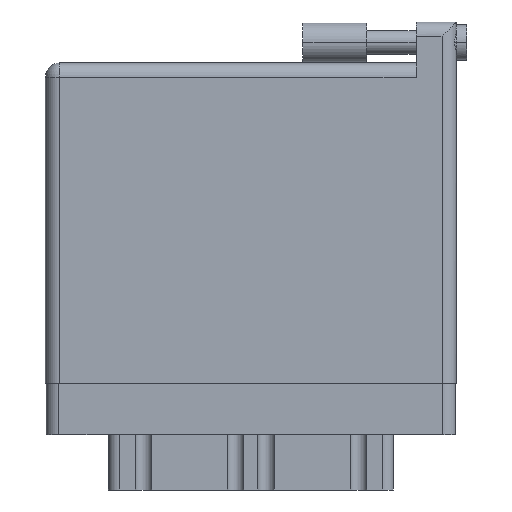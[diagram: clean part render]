
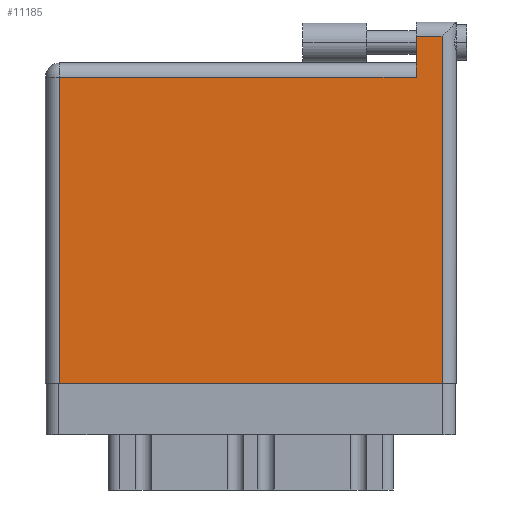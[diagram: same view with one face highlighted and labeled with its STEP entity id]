
A CAD part, front view. The second image highlights one B-rep face of the part: STEP entity #11185.
In plain terms, the highlighted face is planar.
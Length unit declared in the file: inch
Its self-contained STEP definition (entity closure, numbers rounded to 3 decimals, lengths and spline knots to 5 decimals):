
#1038 = CARTESIAN_POINT ( 'NONE',  ( 1.811, 1.496, 0. ) ) ;
#2209 = ORIENTED_EDGE ( 'NONE', *, *, #26951, .T. ) ;
#2925 = LINE ( 'NONE', #11515, #13442 ) ;
#6013 = CARTESIAN_POINT ( 'NONE',  ( 1.938, 1.696, 0. ) ) ;
#7605 = EDGE_CURVE ( 'NONE', #32291, #21695, #13693, .T. ) ;
#8511 = ORIENTED_EDGE ( 'NONE', *, *, #27737, .T. ) ;
#10071 = EDGE_CURVE ( 'NONE', #16131, #33182, #20262, .T. ) ;
#10542 = EDGE_LOOP ( 'NONE', ( #20968, #24654, #11697, #2209, #25558, #8511 ) ) ;
#11185 = ADVANCED_FACE ( 'NONE', ( #16933 ), #34552, .F. ) ;
#11515 = CARTESIAN_POINT ( 'NONE',  ( 1.938, 1.766, 0. ) ) ;
#11697 = ORIENTED_EDGE ( 'NONE', *, *, #7605, .T. ) ;
#12974 = LINE ( 'NONE', #15724, #29293 ) ;
#13442 = VECTOR ( 'NONE', #20741, 39.37008 ) ;
#13495 = DIRECTION ( 'NONE',  ( -1., 0., 0. ) ) ;
#13693 = LINE ( 'NONE', #25437, #14811 ) ;
#13729 = CARTESIAN_POINT ( 'NONE',  ( 1.811, 1.696, 0. ) ) ;
#14811 = VECTOR ( 'NONE', #13495, 39.37008 ) ;
#15724 = CARTESIAN_POINT ( 'NONE',  ( 0., 0., 0. ) ) ;
#16131 = VERTEX_POINT ( 'NONE', #1038 ) ;
#16756 = VECTOR ( 'NONE', #35414, 39.37008 ) ;
#16933 = FACE_OUTER_BOUND ( 'NONE', #10542, .T. ) ;
#17418 = LINE ( 'NONE', #37764, #16756 ) ;
#17727 = CARTESIAN_POINT ( 'NONE',  ( 0., 1.496, 0. ) ) ;
#19081 = VERTEX_POINT ( 'NONE', #27809 ) ;
#19382 = VECTOR ( 'NONE', #32185, 39.37008 ) ;
#20262 = LINE ( 'NONE', #17727, #19382 ) ;
#20741 = DIRECTION ( 'NONE',  ( 0., 1., 0. ) ) ;
#20808 = EDGE_CURVE ( 'NONE', #19081, #32291, #2925, .T. ) ;
#20968 = ORIENTED_EDGE ( 'NONE', *, *, #34785, .T. ) ;
#21695 = VERTEX_POINT ( 'NONE', #13729 ) ;
#22420 = CARTESIAN_POINT ( 'NONE',  ( 0., 1.566, 0. ) ) ;
#22593 = CARTESIAN_POINT ( 'NONE',  ( 0.07, 0., 0. ) ) ;
#24654 = ORIENTED_EDGE ( 'NONE', *, *, #20808, .T. ) ;
#24979 = LINE ( 'NONE', #36921, #34314 ) ;
#25354 = DIRECTION ( 'NONE',  ( 0., 0., -1. ) ) ;
#25437 = CARTESIAN_POINT ( 'NONE',  ( 0., 1.696, 0. ) ) ;
#25558 = ORIENTED_EDGE ( 'NONE', *, *, #10071, .T. ) ;
#26951 = EDGE_CURVE ( 'NONE', #21695, #16131, #17418, .T. ) ;
#27737 = EDGE_CURVE ( 'NONE', #33182, #33279, #24979, .T. ) ;
#27809 = CARTESIAN_POINT ( 'NONE',  ( 1.938, 0., 0. ) ) ;
#29293 = VECTOR ( 'NONE', #36868, 39.37008 ) ;
#32185 = DIRECTION ( 'NONE',  ( -1., 0., 0. ) ) ;
#32291 = VERTEX_POINT ( 'NONE', #6013 ) ;
#33182 = VERTEX_POINT ( 'NONE', #37659 ) ;
#33279 = VERTEX_POINT ( 'NONE', #22593 ) ;
#33973 = DIRECTION ( 'NONE',  ( 0., -1., 0. ) ) ;
#34314 = VECTOR ( 'NONE', #33973, 39.37008 ) ;
#34365 = DIRECTION ( 'NONE',  ( -1., 0., 0. ) ) ;
#34552 = PLANE ( 'NONE',  #35211 ) ;
#34785 = EDGE_CURVE ( 'NONE', #33279, #19081, #12974, .T. ) ;
#35211 = AXIS2_PLACEMENT_3D ( 'NONE', #22420, #25354, #34365 ) ;
#35414 = DIRECTION ( 'NONE',  ( 0., -1., 0. ) ) ;
#36868 = DIRECTION ( 'NONE',  ( 1., 0., 0. ) ) ;
#36921 = CARTESIAN_POINT ( 'NONE',  ( 0.07, 0., 0. ) ) ;
#37659 = CARTESIAN_POINT ( 'NONE',  ( 0.07, 1.496, 0. ) ) ;
#37764 = CARTESIAN_POINT ( 'NONE',  ( 1.811, 1.766, 0. ) ) ;
